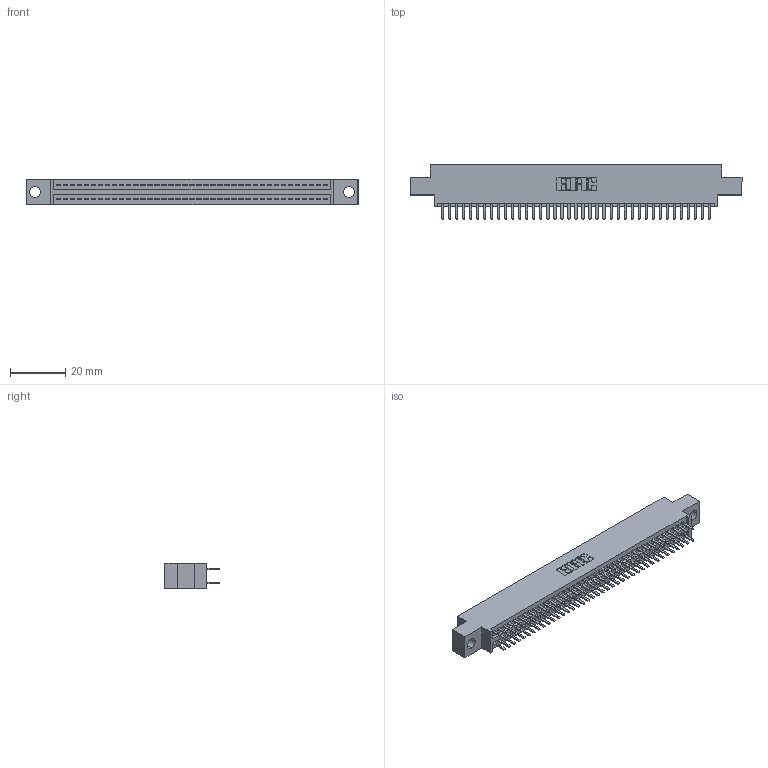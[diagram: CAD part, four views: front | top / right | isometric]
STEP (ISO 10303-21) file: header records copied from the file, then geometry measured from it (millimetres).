
FILE_DESCRIPTION (( 'STEP AP203' ), '1' );
FILE_NAME ('345-078-520-804.STEP', '2018-10-02T19:28:52', ( '' ), ( '' ), 'SwSTEP 2.0', 'SolidWorks 2016', '' );
FILE_SCHEMA (( 'CONFIG_CONTROL_DESIGN' ));
Length unit declared in the file: inch
Products named in the file (3): 345-292-001_345-293-120; 345-078-520-804; 345 Part_0.170 Offset - 0.156 Dia-TH
Assembly tree (79 placements, depth 2):
  345-078-520-804
    345 Part_0.170 Offset - 0.156 Dia-TH
    345-292-001_345-293-120  x78
Bounding box: 120.27 x 19.68 x 9.4 mm (x, y, z)
Volume: 11419.7 mm3; surface area: 16707.8 mm2
Topology: 79 solids, 79 shells, 4342 faces, 12599 edges, 8190 vertices
Faces by surface type: plane 2814, cylinder 1528
Entity records: 31253 total; most frequent: CARTESIAN_POINT 5256, ORIENTED_EDGE 5178, DIRECTION 4625, EDGE_CURVE 2589, LINE 2297, VECTOR 2297, VERTEX_POINT 1722, AXIS2_PLACEMENT_3D 1164
